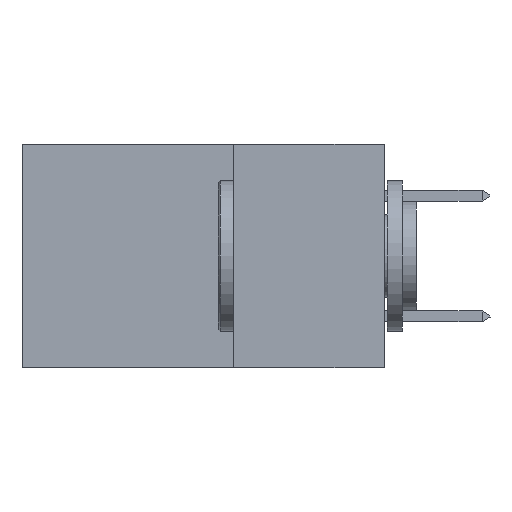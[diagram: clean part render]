
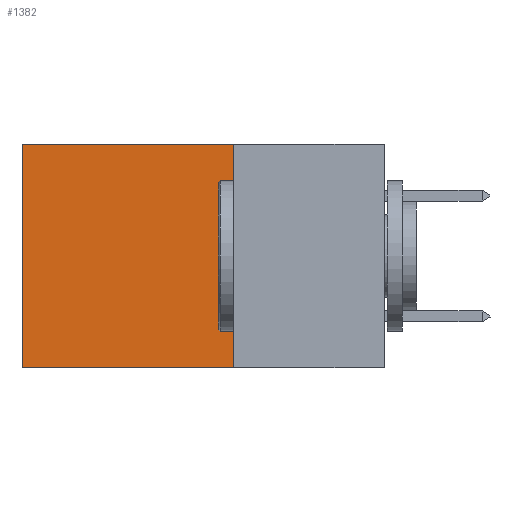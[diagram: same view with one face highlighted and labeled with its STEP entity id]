
A CAD part, left-side view. The second image highlights one B-rep face of the part: STEP entity #1382.
In plain terms, the highlighted planar face has unit normal (-1, 0, 0).
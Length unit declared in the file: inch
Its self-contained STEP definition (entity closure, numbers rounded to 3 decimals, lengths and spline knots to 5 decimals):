
#158 = DIRECTION ( 'NONE',  ( 0., 1., 0. ) ) ;
#306 = EDGE_CURVE ( 'NONE', #12181, #15898, #14378, .T. ) ;
#401 = VECTOR ( 'NONE', #4482, 39.37008 ) ;
#1352 = CARTESIAN_POINT ( 'NONE',  ( 0.2875, 0.25, 0. ) ) ;
#1382 = ADVANCED_FACE ( 'NONE', ( #1884 ), #12993, .F. ) ;
#1428 = VECTOR ( 'NONE', #158, 39.37008 ) ;
#1657 = CARTESIAN_POINT ( 'NONE',  ( 0.2875, 0.6, 0. ) ) ;
#1884 = FACE_OUTER_BOUND ( 'NONE', #14497, .T. ) ;
#2583 = VECTOR ( 'NONE', #16004, 39.37008 ) ;
#3287 = CARTESIAN_POINT ( 'NONE',  ( 0.2875, 0.25, -0.37 ) ) ;
#3374 = CARTESIAN_POINT ( 'NONE',  ( 0.2875, 0.25, 0. ) ) ;
#4366 = DIRECTION ( 'NONE',  ( 0., 0., -1. ) ) ;
#4482 = DIRECTION ( 'NONE',  ( 0., 0., -1. ) ) ;
#4907 = EDGE_CURVE ( 'NONE', #6207, #11988, #11309, .T. ) ;
#6081 = ORIENTED_EDGE ( 'NONE', *, *, #306, .F. ) ;
#6146 = LINE ( 'NONE', #15976, #401 ) ;
#6207 = VERTEX_POINT ( 'NONE', #1352 ) ;
#7110 = AXIS2_PLACEMENT_3D ( 'NONE', #3374, #15001, #7633 ) ;
#7633 = DIRECTION ( 'NONE',  ( 0., 0., -1. ) ) ;
#8341 = CARTESIAN_POINT ( 'NONE',  ( 0.2875, 0.25, 0. ) ) ;
#8417 = VECTOR ( 'NONE', #4366, 39.37008 ) ;
#8902 = CARTESIAN_POINT ( 'NONE',  ( 0.2875, 0.25, -0.37 ) ) ;
#9477 = EDGE_CURVE ( 'NONE', #11988, #15898, #12020, .T. ) ;
#9837 = EDGE_CURVE ( 'NONE', #6207, #12181, #6146, .T. ) ;
#10315 = ORIENTED_EDGE ( 'NONE', *, *, #4907, .T. ) ;
#10608 = CARTESIAN_POINT ( 'NONE',  ( 0.2875, 0.6, -0.37 ) ) ;
#11309 = LINE ( 'NONE', #8341, #1428 ) ;
#11988 = VERTEX_POINT ( 'NONE', #14726 ) ;
#12020 = LINE ( 'NONE', #1657, #8417 ) ;
#12181 = VERTEX_POINT ( 'NONE', #3287 ) ;
#12330 = ORIENTED_EDGE ( 'NONE', *, *, #9477, .T. ) ;
#12901 = ORIENTED_EDGE ( 'NONE', *, *, #9837, .F. ) ;
#12993 = PLANE ( 'NONE',  #7110 ) ;
#14378 = LINE ( 'NONE', #8902, #2583 ) ;
#14497 = EDGE_LOOP ( 'NONE', ( #12330, #6081, #12901, #10315 ) ) ;
#14726 = CARTESIAN_POINT ( 'NONE',  ( 0.2875, 0.6, 0. ) ) ;
#15001 = DIRECTION ( 'NONE',  ( 1., 0., 0. ) ) ;
#15898 = VERTEX_POINT ( 'NONE', #10608 ) ;
#15976 = CARTESIAN_POINT ( 'NONE',  ( 0.2875, 0.25, 0. ) ) ;
#16004 = DIRECTION ( 'NONE',  ( 0., 1., 0. ) ) ;
